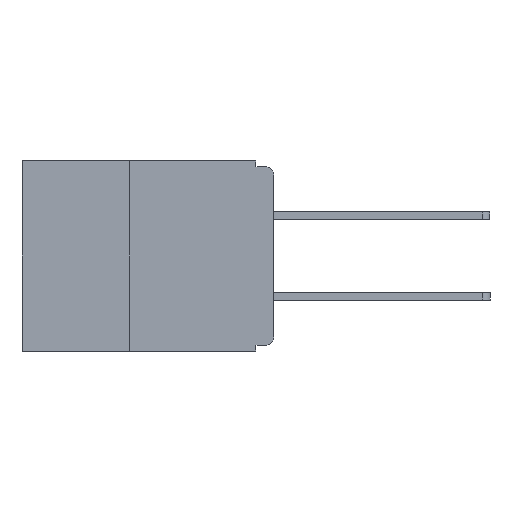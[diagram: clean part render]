
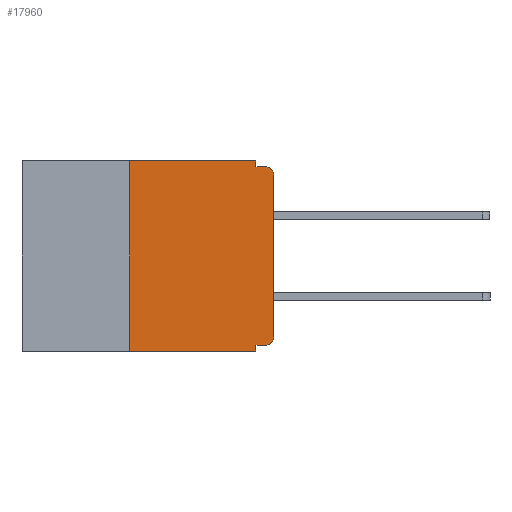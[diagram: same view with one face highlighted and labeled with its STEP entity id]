
A CAD part, left-side view. The second image highlights one B-rep face of the part: STEP entity #17960.
In plain terms, the highlighted planar face has unit normal (-1, 0, 0).
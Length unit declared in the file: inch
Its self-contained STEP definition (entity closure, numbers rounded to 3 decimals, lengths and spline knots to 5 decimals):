
#151 = CARTESIAN_POINT ( 'NONE',  ( 0., 0., -0.01 ) ) ;
#190 = AXIS2_PLACEMENT_3D ( 'NONE', #253, #12286, #2006 ) ;
#253 = CARTESIAN_POINT ( 'NONE',  ( 0., 0.015, -0.305 ) ) ;
#741 = VERTEX_POINT ( 'NONE', #5394 ) ;
#746 = VECTOR ( 'NONE', #15180, 39.37008 ) ;
#1405 = CARTESIAN_POINT ( 'NONE',  ( 0., 0.031, 0. ) ) ;
#2006 = DIRECTION ( 'NONE',  ( 0., 0., -1. ) ) ;
#2415 = VECTOR ( 'NONE', #20791, 39.37008 ) ;
#2588 = CARTESIAN_POINT ( 'NONE',  ( 0., 0.031, -0.33 ) ) ;
#2767 = DIRECTION ( 'NONE',  ( 0., 0., -1. ) ) ;
#2952 = LINE ( 'NONE', #6477, #16075 ) ;
#3193 = CARTESIAN_POINT ( 'NONE',  ( 0., 0.031, 0. ) ) ;
#3872 = EDGE_CURVE ( 'NONE', #4634, #14893, #6497, .T. ) ;
#3939 = DIRECTION ( 'NONE',  ( -1., 0., 0. ) ) ;
#4634 = VERTEX_POINT ( 'NONE', #6568 ) ;
#5394 = CARTESIAN_POINT ( 'NONE',  ( 0., 0.015, -0.01 ) ) ;
#5795 = EDGE_CURVE ( 'NONE', #6853, #17485, #13362, .T. ) ;
#6251 = CARTESIAN_POINT ( 'NONE',  ( 0., 0., -0.305 ) ) ;
#6477 = CARTESIAN_POINT ( 'NONE',  ( 0., 0.437, 0. ) ) ;
#6497 = LINE ( 'NONE', #21876, #20197 ) ;
#6568 = CARTESIAN_POINT ( 'NONE',  ( 0., 0.25, -0.33 ) ) ;
#6692 = CIRCLE ( 'NONE', #190, 0.015 ) ;
#6853 = VERTEX_POINT ( 'NONE', #20588 ) ;
#6981 = EDGE_CURVE ( 'NONE', #4634, #17485, #8273, .T. ) ;
#7263 = CARTESIAN_POINT ( 'NONE',  ( 0., 0., -0.32 ) ) ;
#7534 = LINE ( 'NONE', #151, #2415 ) ;
#8024 = EDGE_LOOP ( 'NONE', ( #18531, #18649, #18902, #19001, #19248, #19308, #19506, #19524, #19630, #19673 ) ) ;
#8273 = LINE ( 'NONE', #19200, #16853 ) ;
#8988 = DIRECTION ( 'NONE',  ( 0., 1., 0. ) ) ;
#9403 = EDGE_CURVE ( 'NONE', #14363, #6853, #21496, .T. ) ;
#9536 = DIRECTION ( 'NONE',  ( 1., 0., 0. ) ) ;
#9711 = VERTEX_POINT ( 'NONE', #3193 ) ;
#9946 = LINE ( 'NONE', #1405, #746 ) ;
#11168 = CARTESIAN_POINT ( 'NONE',  ( 0., 0.437, 0. ) ) ;
#11878 = VERTEX_POINT ( 'NONE', #6251 ) ;
#11888 = AXIS2_PLACEMENT_3D ( 'NONE', #11168, #9536, #21460 ) ;
#12286 = DIRECTION ( 'NONE',  ( -1., 0., 0. ) ) ;
#12746 = FACE_OUTER_BOUND ( 'NONE', #8024, .T. ) ;
#12829 = EDGE_CURVE ( 'NONE', #14757, #741, #17788, .T. ) ;
#13251 = EDGE_CURVE ( 'NONE', #11878, #14757, #14249, .T. ) ;
#13362 = LINE ( 'NONE', #2588, #13891 ) ;
#13891 = VECTOR ( 'NONE', #2767, 39.37008 ) ;
#14217 = CARTESIAN_POINT ( 'NONE',  ( 0., 0.015, -0.025 ) ) ;
#14249 = LINE ( 'NONE', #17013, #18337 ) ;
#14363 = VERTEX_POINT ( 'NONE', #16733 ) ;
#14489 = CARTESIAN_POINT ( 'NONE',  ( 0., 0.031, -0.01 ) ) ;
#14687 = VERTEX_POINT ( 'NONE', #14489 ) ;
#14757 = VERTEX_POINT ( 'NONE', #18145 ) ;
#14893 = VERTEX_POINT ( 'NONE', #21863 ) ;
#15180 = DIRECTION ( 'NONE',  ( 0., 0., -1. ) ) ;
#15935 = DIRECTION ( 'NONE',  ( 0., 0., -1. ) ) ;
#16075 = VECTOR ( 'NONE', #18498, 39.37008 ) ;
#16093 = EDGE_CURVE ( 'NONE', #9711, #14687, #9946, .T. ) ;
#16254 = EDGE_CURVE ( 'NONE', #14363, #11878, #6692, .T. ) ;
#16733 = CARTESIAN_POINT ( 'NONE',  ( 0., 0.015, -0.32 ) ) ;
#16853 = VECTOR ( 'NONE', #19162, 39.37008 ) ;
#17007 = VECTOR ( 'NONE', #8988, 39.37008 ) ;
#17013 = CARTESIAN_POINT ( 'NONE',  ( 0., 0., 0. ) ) ;
#17097 = DIRECTION ( 'NONE',  ( 0., 0., 1. ) ) ;
#17485 = VERTEX_POINT ( 'NONE', #20282 ) ;
#17788 = CIRCLE ( 'NONE', #18461, 0.015 ) ;
#17960 = ADVANCED_FACE ( 'NONE', ( #12746 ), #19817, .F. ) ;
#18145 = CARTESIAN_POINT ( 'NONE',  ( 0., 0., -0.025 ) ) ;
#18337 = VECTOR ( 'NONE', #17097, 39.37008 ) ;
#18461 = AXIS2_PLACEMENT_3D ( 'NONE', #14217, #3939, #15935 ) ;
#18498 = DIRECTION ( 'NONE',  ( 0., -1., 0. ) ) ;
#18531 = ORIENTED_EDGE ( 'NONE', *, *, #13251, .T. ) ;
#18649 = ORIENTED_EDGE ( 'NONE', *, *, #12829, .T. ) ;
#18902 = ORIENTED_EDGE ( 'NONE', *, *, #21261, .F. ) ;
#19001 = ORIENTED_EDGE ( 'NONE', *, *, #16093, .F. ) ;
#19162 = DIRECTION ( 'NONE',  ( 0., -1., 0. ) ) ;
#19200 = CARTESIAN_POINT ( 'NONE',  ( 0., 0.437, -0.33 ) ) ;
#19248 = ORIENTED_EDGE ( 'NONE', *, *, #21665, .F. ) ;
#19308 = ORIENTED_EDGE ( 'NONE', *, *, #3872, .F. ) ;
#19506 = ORIENTED_EDGE ( 'NONE', *, *, #6981, .T. ) ;
#19524 = ORIENTED_EDGE ( 'NONE', *, *, #5795, .F. ) ;
#19630 = ORIENTED_EDGE ( 'NONE', *, *, #9403, .F. ) ;
#19673 = ORIENTED_EDGE ( 'NONE', *, *, #16254, .T. ) ;
#19817 = PLANE ( 'NONE',  #11888 ) ;
#20197 = VECTOR ( 'NONE', #21902, 39.37008 ) ;
#20282 = CARTESIAN_POINT ( 'NONE',  ( 0., 0.031, -0.33 ) ) ;
#20588 = CARTESIAN_POINT ( 'NONE',  ( 0., 0.031, -0.32 ) ) ;
#20791 = DIRECTION ( 'NONE',  ( 0., -1., 0. ) ) ;
#21261 = EDGE_CURVE ( 'NONE', #14687, #741, #7534, .T. ) ;
#21460 = DIRECTION ( 'NONE',  ( 0., 0., -1. ) ) ;
#21496 = LINE ( 'NONE', #7263, #17007 ) ;
#21665 = EDGE_CURVE ( 'NONE', #14893, #9711, #2952, .T. ) ;
#21863 = CARTESIAN_POINT ( 'NONE',  ( 0., 0.25, 0. ) ) ;
#21876 = CARTESIAN_POINT ( 'NONE',  ( 0., 0.25, -0.33 ) ) ;
#21902 = DIRECTION ( 'NONE',  ( 0., 0., 1. ) ) ;
